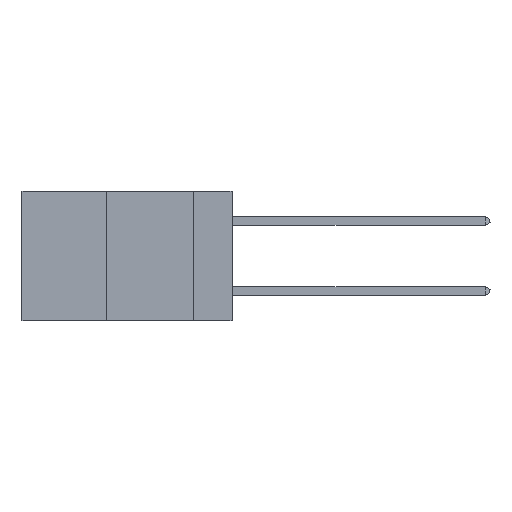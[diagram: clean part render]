
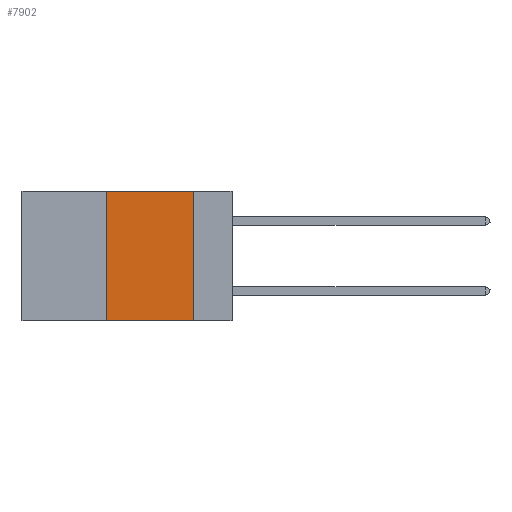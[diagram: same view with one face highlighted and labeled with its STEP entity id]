
A CAD part, left-side view. The second image highlights one B-rep face of the part: STEP entity #7902.
In plain terms, the highlighted planar face has unit normal (-1, 0, 0).
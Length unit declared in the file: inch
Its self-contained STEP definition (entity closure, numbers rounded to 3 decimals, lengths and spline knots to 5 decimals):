
#256 = VERTEX_POINT ( 'NONE', #12827 ) ;
#263 = CARTESIAN_POINT ( 'NONE',  ( 0., 0.6, 0. ) ) ;
#1332 = EDGE_LOOP ( 'NONE', ( #22640, #13789, #21559, #8570 ) ) ;
#2287 = DIRECTION ( 'NONE',  ( 0., -1., 0. ) ) ;
#3138 = VERTEX_POINT ( 'NONE', #12041 ) ;
#3912 = VECTOR ( 'NONE', #2287, 39.37008 ) ;
#4325 = VECTOR ( 'NONE', #23324, 39.37008 ) ;
#5938 = EDGE_CURVE ( 'NONE', #3138, #9453, #9431, .T. ) ;
#6047 = CARTESIAN_POINT ( 'NONE',  ( 0., 0.36, -0.37 ) ) ;
#7575 = LINE ( 'NONE', #14076, #16897 ) ;
#7902 = ADVANCED_FACE ( 'NONE', ( #17197 ), #19205, .F. ) ;
#7909 = AXIS2_PLACEMENT_3D ( 'NONE', #263, #21050, #10015 ) ;
#8086 = EDGE_CURVE ( 'NONE', #9453, #256, #7575, .T. ) ;
#8557 = CARTESIAN_POINT ( 'NONE',  ( 0., 0.6, 0. ) ) ;
#8570 = ORIENTED_EDGE ( 'NONE', *, *, #17263, .T. ) ;
#8868 = VECTOR ( 'NONE', #15480, 39.37008 ) ;
#9431 = LINE ( 'NONE', #8557, #4325 ) ;
#9453 = VERTEX_POINT ( 'NONE', #14503 ) ;
#10015 = DIRECTION ( 'NONE',  ( 0., 0., -1. ) ) ;
#12041 = CARTESIAN_POINT ( 'NONE',  ( 0., 0.36, 0. ) ) ;
#12567 = VERTEX_POINT ( 'NONE', #6047 ) ;
#12827 = CARTESIAN_POINT ( 'NONE',  ( 0., 0.11, -0.37 ) ) ;
#13647 = CARTESIAN_POINT ( 'NONE',  ( 0., 0.36, 0. ) ) ;
#13695 = CARTESIAN_POINT ( 'NONE',  ( 0., 0.6, -0.37 ) ) ;
#13789 = ORIENTED_EDGE ( 'NONE', *, *, #5938, .F. ) ;
#13979 = LINE ( 'NONE', #13695, #3912 ) ;
#14076 = CARTESIAN_POINT ( 'NONE',  ( 0., 0.11, 0. ) ) ;
#14503 = CARTESIAN_POINT ( 'NONE',  ( 0., 0.11, 0. ) ) ;
#15480 = DIRECTION ( 'NONE',  ( 0., 0., 1. ) ) ;
#16897 = VECTOR ( 'NONE', #21517, 39.37008 ) ;
#17197 = FACE_OUTER_BOUND ( 'NONE', #1332, .T. ) ;
#17263 = EDGE_CURVE ( 'NONE', #12567, #256, #13979, .T. ) ;
#19205 = PLANE ( 'NONE',  #7909 ) ;
#19856 = LINE ( 'NONE', #13647, #8868 ) ;
#20938 = EDGE_CURVE ( 'NONE', #12567, #3138, #19856, .T. ) ;
#21050 = DIRECTION ( 'NONE',  ( 1., 0., 0. ) ) ;
#21517 = DIRECTION ( 'NONE',  ( 0., 0., -1. ) ) ;
#21559 = ORIENTED_EDGE ( 'NONE', *, *, #20938, .F. ) ;
#22640 = ORIENTED_EDGE ( 'NONE', *, *, #8086, .F. ) ;
#23324 = DIRECTION ( 'NONE',  ( 0., -1., 0. ) ) ;
